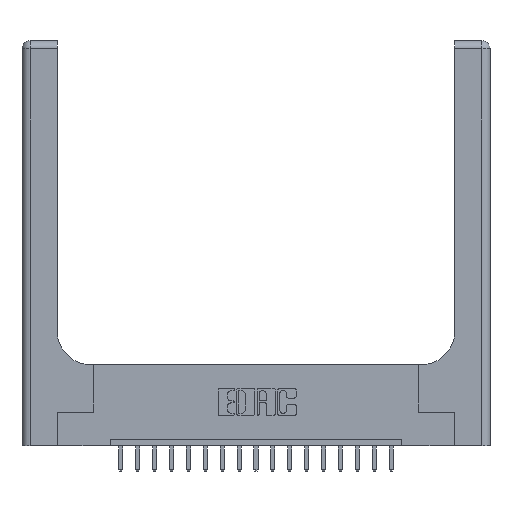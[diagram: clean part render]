
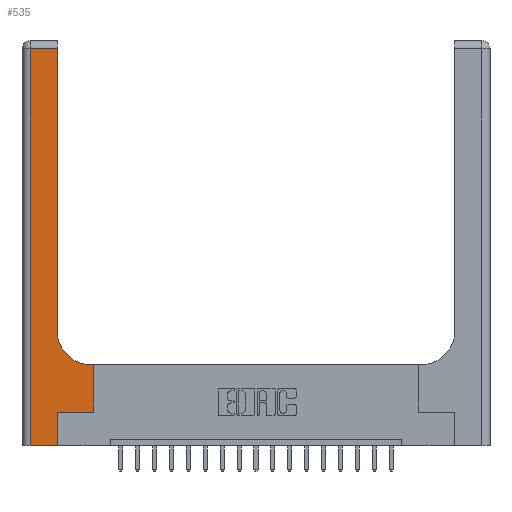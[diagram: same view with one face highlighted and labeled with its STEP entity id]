
A CAD part, top view. The second image highlights one B-rep face of the part: STEP entity #535.
In plain terms, the highlighted planar face has unit normal (0, 0, 1).
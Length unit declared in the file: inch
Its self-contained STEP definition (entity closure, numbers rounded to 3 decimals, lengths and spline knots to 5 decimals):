
#460 = EDGE_CURVE ( 'NONE', #11497, #16090, #16994, .T. ) ;
#535 = ADVANCED_FACE ( 'NONE', ( #18499 ), #4764, .F. ) ;
#762 = VERTEX_POINT ( 'NONE', #15091 ) ;
#918 = EDGE_CURVE ( 'NONE', #10677, #7309, #9616, .T. ) ;
#936 = CARTESIAN_POINT ( 'NONE',  ( 0., 2.94, 0.37 ) ) ;
#1482 = CARTESIAN_POINT ( 'NONE',  ( 0.26, 3., 0.37 ) ) ;
#1743 = EDGE_CURVE ( 'NONE', #762, #7405, #7848, .T. ) ;
#1895 = LINE ( 'NONE', #14026, #13334 ) ;
#2194 = EDGE_CURVE ( 'NONE', #7405, #3588, #18668, .T. ) ;
#2227 = ORIENTED_EDGE ( 'NONE', *, *, #13970, .T. ) ;
#2898 = LINE ( 'NONE', #18407, #14975 ) ;
#3238 = DIRECTION ( 'NONE',  ( 0., -1., 0. ) ) ;
#3287 = DIRECTION ( 'NONE',  ( -1., 0., 0. ) ) ;
#3437 = CARTESIAN_POINT ( 'NONE',  ( 0.528, 0.25, 0.37 ) ) ;
#3553 = CARTESIAN_POINT ( 'NONE',  ( 0.265, 0., 0.37 ) ) ;
#3588 = VERTEX_POINT ( 'NONE', #11807 ) ;
#3718 = LINE ( 'NONE', #936, #16641 ) ;
#3960 = VERTEX_POINT ( 'NONE', #17559 ) ;
#4479 = DIRECTION ( 'NONE',  ( 0., 0., -1. ) ) ;
#4764 = PLANE ( 'NONE',  #11304 ) ;
#5169 = DIRECTION ( 'NONE',  ( 1., 0., 0. ) ) ;
#5703 = CARTESIAN_POINT ( 'NONE',  ( 0.51, 0.85, 0.37 ) ) ;
#6747 = ORIENTED_EDGE ( 'NONE', *, *, #1743, .T. ) ;
#6771 = ORIENTED_EDGE ( 'NONE', *, *, #918, .T. ) ;
#7309 = VERTEX_POINT ( 'NONE', #7926 ) ;
#7405 = VERTEX_POINT ( 'NONE', #9618 ) ;
#7714 = LINE ( 'NONE', #15083, #15526 ) ;
#7754 = DIRECTION ( 'NONE',  ( -1., 0., 0. ) ) ;
#7848 = LINE ( 'NONE', #13913, #8783 ) ;
#7926 = CARTESIAN_POINT ( 'NONE',  ( 0.528, 0.6, 0.37 ) ) ;
#8143 = VECTOR ( 'NONE', #10926, 39.37008 ) ;
#8783 = VECTOR ( 'NONE', #5169, 39.37008 ) ;
#9063 = ORIENTED_EDGE ( 'NONE', *, *, #10801, .T. ) ;
#9426 = CARTESIAN_POINT ( 'NONE',  ( 0., 3., 0.37 ) ) ;
#9616 = LINE ( 'NONE', #3437, #17995 ) ;
#9618 = CARTESIAN_POINT ( 'NONE',  ( 0.265, 0., 0.37 ) ) ;
#10228 = CARTESIAN_POINT ( 'NONE',  ( 0.528, 0.25, 0.37 ) ) ;
#10383 = VERTEX_POINT ( 'NONE', #12148 ) ;
#10387 = VECTOR ( 'NONE', #17282, 39.37008 ) ;
#10677 = VERTEX_POINT ( 'NONE', #10228 ) ;
#10801 = EDGE_CURVE ( 'NONE', #3960, #762, #7714, .T. ) ;
#10926 = DIRECTION ( 'NONE',  ( 0., 1., 0. ) ) ;
#11304 = AXIS2_PLACEMENT_3D ( 'NONE', #9426, #4479, #7754 ) ;
#11497 = VERTEX_POINT ( 'NONE', #12355 ) ;
#11807 = CARTESIAN_POINT ( 'NONE',  ( 0.265, 0.25, 0.37 ) ) ;
#11951 = EDGE_CURVE ( 'NONE', #7309, #10383, #1895, .T. ) ;
#12104 = ORIENTED_EDGE ( 'NONE', *, *, #460, .T. ) ;
#12148 = CARTESIAN_POINT ( 'NONE',  ( 0.51, 0.6, 0.37 ) ) ;
#12310 = EDGE_CURVE ( 'NONE', #10383, #11497, #16391, .T. ) ;
#12355 = CARTESIAN_POINT ( 'NONE',  ( 0.26, 0.85, 0.37 ) ) ;
#12899 = AXIS2_PLACEMENT_3D ( 'NONE', #5703, #19050, #19238 ) ;
#13334 = VECTOR ( 'NONE', #3287, 39.37008 ) ;
#13822 = DIRECTION ( 'NONE',  ( 1., 0., 0. ) ) ;
#13913 = CARTESIAN_POINT ( 'NONE',  ( 0., 0., 0.37 ) ) ;
#13970 = EDGE_CURVE ( 'NONE', #3588, #10677, #2898, .T. ) ;
#14026 = CARTESIAN_POINT ( 'NONE',  ( 0.26, 0.6, 0.37 ) ) ;
#14067 = EDGE_LOOP ( 'NONE', ( #12104, #15909, #9063, #6747, #14610, #2227, #6771, #17681, #15629 ) ) ;
#14610 = ORIENTED_EDGE ( 'NONE', *, *, #2194, .T. ) ;
#14975 = VECTOR ( 'NONE', #13822, 39.37008 ) ;
#15083 = CARTESIAN_POINT ( 'NONE',  ( 0.06, 3., 0.37 ) ) ;
#15091 = CARTESIAN_POINT ( 'NONE',  ( 0.06, 0., 0.37 ) ) ;
#15526 = VECTOR ( 'NONE', #3238, 39.37008 ) ;
#15629 = ORIENTED_EDGE ( 'NONE', *, *, #12310, .T. ) ;
#15909 = ORIENTED_EDGE ( 'NONE', *, *, #18863, .T. ) ;
#16090 = VERTEX_POINT ( 'NONE', #16345 ) ;
#16345 = CARTESIAN_POINT ( 'NONE',  ( 0.26, 2.94, 0.37 ) ) ;
#16391 = CIRCLE ( 'NONE', #12899, 0.25 ) ;
#16641 = VECTOR ( 'NONE', #19146, 39.37008 ) ;
#16994 = LINE ( 'NONE', #1482, #8143 ) ;
#17282 = DIRECTION ( 'NONE',  ( 0., 1., 0. ) ) ;
#17559 = CARTESIAN_POINT ( 'NONE',  ( 0.06, 2.94, 0.37 ) ) ;
#17681 = ORIENTED_EDGE ( 'NONE', *, *, #11951, .T. ) ;
#17995 = VECTOR ( 'NONE', #18566, 39.37008 ) ;
#18407 = CARTESIAN_POINT ( 'NONE',  ( 0.265, 0.25, 0.37 ) ) ;
#18499 = FACE_OUTER_BOUND ( 'NONE', #14067, .T. ) ;
#18566 = DIRECTION ( 'NONE',  ( 0., 1., 0. ) ) ;
#18668 = LINE ( 'NONE', #3553, #10387 ) ;
#18863 = EDGE_CURVE ( 'NONE', #16090, #3960, #3718, .T. ) ;
#19050 = DIRECTION ( 'NONE',  ( 0., 0., -1. ) ) ;
#19146 = DIRECTION ( 'NONE',  ( -1., 0., 0. ) ) ;
#19238 = DIRECTION ( 'NONE',  ( 1., 0., 0. ) ) ;
